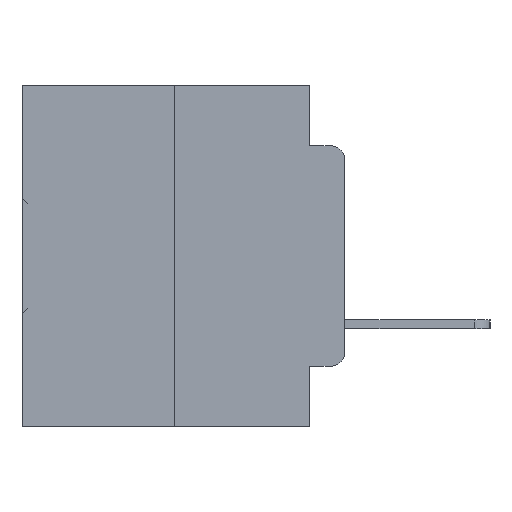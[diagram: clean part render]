
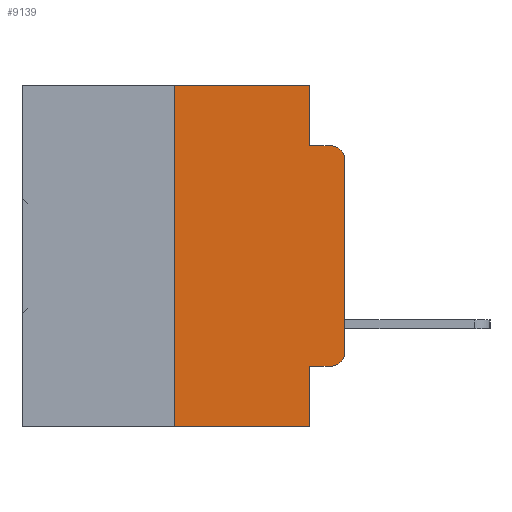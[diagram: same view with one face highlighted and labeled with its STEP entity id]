
A CAD part, left-side view. The second image highlights one B-rep face of the part: STEP entity #9139.
In plain terms, the highlighted planar face has unit normal (-1, 0, 0).
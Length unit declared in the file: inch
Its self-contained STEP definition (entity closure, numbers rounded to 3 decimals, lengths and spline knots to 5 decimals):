
#1563 = VERTEX_POINT ( 'NONE', #1851 ) ;
#1601 = VECTOR ( 'NONE', #23980, 39.37008 ) ;
#1741 = LINE ( 'NONE', #18647, #15443 ) ;
#1851 = CARTESIAN_POINT ( 'NONE',  ( 0., 0.25, 0. ) ) ;
#2035 = CARTESIAN_POINT ( 'NONE',  ( 0., 0.25, -0.5 ) ) ;
#2182 = CIRCLE ( 'NONE', #25919, 0.02 ) ;
#2193 = ORIENTED_EDGE ( 'NONE', *, *, #5478, .T. ) ;
#2387 = DIRECTION ( 'NONE',  ( 0., -1., 0. ) ) ;
#2724 = VERTEX_POINT ( 'NONE', #26883 ) ;
#2947 = VERTEX_POINT ( 'NONE', #3113 ) ;
#3001 = LINE ( 'NONE', #33258, #28991 ) ;
#3113 = CARTESIAN_POINT ( 'NONE',  ( 0., 0.051, -0.4115 ) ) ;
#3848 = DIRECTION ( 'NONE',  ( 0., 0., 1. ) ) ;
#4286 = VECTOR ( 'NONE', #34324, 39.37008 ) ;
#4321 = VERTEX_POINT ( 'NONE', #33627 ) ;
#4866 = LINE ( 'NONE', #33942, #11280 ) ;
#4875 = CARTESIAN_POINT ( 'NONE',  ( 0., 0.473, -0.5 ) ) ;
#5203 = CARTESIAN_POINT ( 'NONE',  ( 0., 0.051, 0. ) ) ;
#5478 = EDGE_CURVE ( 'NONE', #8629, #31810, #34239, .T. ) ;
#6752 = DIRECTION ( 'NONE',  ( 0., -1., 0. ) ) ;
#6924 = ORIENTED_EDGE ( 'NONE', *, *, #15072, .T. ) ;
#7601 = ORIENTED_EDGE ( 'NONE', *, *, #18809, .T. ) ;
#7941 = CARTESIAN_POINT ( 'NONE',  ( 0., 0.473, 0. ) ) ;
#8086 = LINE ( 'NONE', #5203, #1601 ) ;
#8629 = VERTEX_POINT ( 'NONE', #9396 ) ;
#8861 = PLANE ( 'NONE',  #18748 ) ;
#9139 = ADVANCED_FACE ( 'NONE', ( #26643 ), #8861, .F. ) ;
#9396 = CARTESIAN_POINT ( 'NONE',  ( 0., 0., -0.3915 ) ) ;
#11280 = VECTOR ( 'NONE', #31445, 39.37008 ) ;
#11824 = CARTESIAN_POINT ( 'NONE',  ( 0., 0.051, -0.0885 ) ) ;
#13118 = CARTESIAN_POINT ( 'NONE',  ( 0., 0.02, -0.1085 ) ) ;
#13472 = EDGE_CURVE ( 'NONE', #26511, #8629, #2182, .T. ) ;
#14327 = DIRECTION ( 'NONE',  ( 1., 0., 0. ) ) ;
#15072 = EDGE_CURVE ( 'NONE', #29453, #31834, #22834, .T. ) ;
#15443 = VECTOR ( 'NONE', #2387, 39.37008 ) ;
#15797 = DIRECTION ( 'NONE',  ( 0., 0., -1. ) ) ;
#16305 = CARTESIAN_POINT ( 'NONE',  ( 0., 0.02, -0.3915 ) ) ;
#17093 = ORIENTED_EDGE ( 'NONE', *, *, #34649, .T. ) ;
#17801 = CARTESIAN_POINT ( 'NONE',  ( 0., 0.051, -0.5 ) ) ;
#18203 = VECTOR ( 'NONE', #23973, 39.37008 ) ;
#18576 = CARTESIAN_POINT ( 'NONE',  ( 0., 0.25, 0. ) ) ;
#18647 = CARTESIAN_POINT ( 'NONE',  ( 0., 0.051, -0.4115 ) ) ;
#18675 = ORIENTED_EDGE ( 'NONE', *, *, #24819, .F. ) ;
#18748 = AXIS2_PLACEMENT_3D ( 'NONE', #19558, #14327, #32748 ) ;
#18809 = EDGE_CURVE ( 'NONE', #2947, #26511, #1741, .T. ) ;
#18982 = DIRECTION ( 'NONE',  ( 0., 0., -1. ) ) ;
#19509 = LINE ( 'NONE', #18576, #4286 ) ;
#19558 = CARTESIAN_POINT ( 'NONE',  ( 0., 0.473, 0. ) ) ;
#20281 = VECTOR ( 'NONE', #3848, 39.37008 ) ;
#20593 = EDGE_CURVE ( 'NONE', #2947, #31834, #8086, .T. ) ;
#20735 = CIRCLE ( 'NONE', #33959, 0.02 ) ;
#21008 = DIRECTION ( 'NONE',  ( 0., -1., 0. ) ) ;
#22331 = ORIENTED_EDGE ( 'NONE', *, *, #13472, .T. ) ;
#22834 = LINE ( 'NONE', #4875, #28173 ) ;
#23809 = EDGE_LOOP ( 'NONE', ( #2193, #17093, #26170, #34749, #18675, #29886, #6924, #25159, #7601, #22331 ) ) ;
#23820 = VERTEX_POINT ( 'NONE', #11824 ) ;
#23973 = DIRECTION ( 'NONE',  ( 0., -1., 0. ) ) ;
#23980 = DIRECTION ( 'NONE',  ( 0., 0., -1. ) ) ;
#24129 = EDGE_CURVE ( 'NONE', #29453, #1563, #19509, .T. ) ;
#24819 = EDGE_CURVE ( 'NONE', #1563, #4321, #25223, .T. ) ;
#25159 = ORIENTED_EDGE ( 'NONE', *, *, #20593, .F. ) ;
#25223 = LINE ( 'NONE', #7941, #18203 ) ;
#25648 = CARTESIAN_POINT ( 'NONE',  ( 0., 0., -0.1085 ) ) ;
#25919 = AXIS2_PLACEMENT_3D ( 'NONE', #16305, #34718, #18982 ) ;
#26170 = ORIENTED_EDGE ( 'NONE', *, *, #31171, .F. ) ;
#26511 = VERTEX_POINT ( 'NONE', #29734 ) ;
#26643 = FACE_OUTER_BOUND ( 'NONE', #23809, .T. ) ;
#26883 = CARTESIAN_POINT ( 'NONE',  ( 0., 0.02, -0.0885 ) ) ;
#27969 = CARTESIAN_POINT ( 'NONE',  ( 0., 0., 0. ) ) ;
#28173 = VECTOR ( 'NONE', #21008, 39.37008 ) ;
#28991 = VECTOR ( 'NONE', #6752, 39.37008 ) ;
#29407 = EDGE_CURVE ( 'NONE', #4321, #23820, #4866, .T. ) ;
#29453 = VERTEX_POINT ( 'NONE', #2035 ) ;
#29734 = CARTESIAN_POINT ( 'NONE',  ( 0., 0.02, -0.4115 ) ) ;
#29886 = ORIENTED_EDGE ( 'NONE', *, *, #24129, .F. ) ;
#31171 = EDGE_CURVE ( 'NONE', #23820, #2724, #3001, .T. ) ;
#31445 = DIRECTION ( 'NONE',  ( 0., 0., -1. ) ) ;
#31587 = DIRECTION ( 'NONE',  ( -1., 0., 0. ) ) ;
#31810 = VERTEX_POINT ( 'NONE', #25648 ) ;
#31834 = VERTEX_POINT ( 'NONE', #17801 ) ;
#32748 = DIRECTION ( 'NONE',  ( 0., 0., -1. ) ) ;
#33258 = CARTESIAN_POINT ( 'NONE',  ( 0., 0.051, -0.0885 ) ) ;
#33627 = CARTESIAN_POINT ( 'NONE',  ( 0., 0.051, 0. ) ) ;
#33942 = CARTESIAN_POINT ( 'NONE',  ( 0., 0.051, 0. ) ) ;
#33959 = AXIS2_PLACEMENT_3D ( 'NONE', #13118, #31587, #15797 ) ;
#34239 = LINE ( 'NONE', #27969, #20281 ) ;
#34324 = DIRECTION ( 'NONE',  ( 0., 0., 1. ) ) ;
#34649 = EDGE_CURVE ( 'NONE', #31810, #2724, #20735, .T. ) ;
#34718 = DIRECTION ( 'NONE',  ( -1., 0., 0. ) ) ;
#34749 = ORIENTED_EDGE ( 'NONE', *, *, #29407, .F. ) ;
